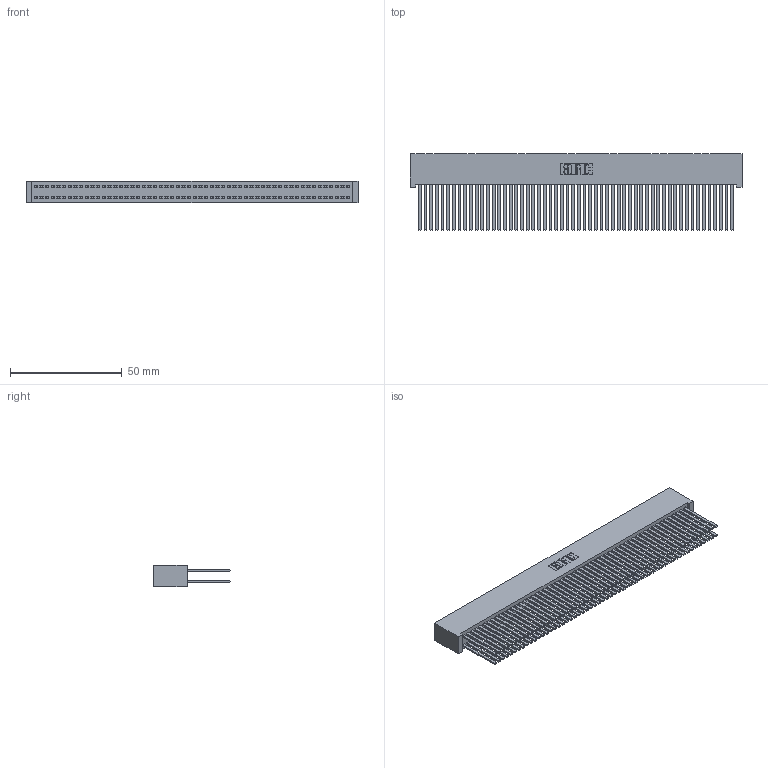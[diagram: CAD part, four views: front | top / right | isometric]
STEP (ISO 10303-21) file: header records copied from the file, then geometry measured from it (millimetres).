
FILE_DESCRIPTION (( 'STEP AP203' ), '1' );
FILE_NAME ('342-112-544-201.STEP', '2018-08-14T12:18:39', ( '' ), ( '' ), 'SwSTEP 2.0', 'SolidWorks 2016', '' );
FILE_SCHEMA (( 'CONFIG_CONTROL_DESIGN' ));
Length unit declared in the file: inch
Products named in the file (3): 345-292-001_345-293-144; 342-112-544-201; 342 Part_Lugless
Assembly tree (113 placements, depth 2):
  342-112-544-201
    342 Part_Lugless
    345-292-001_345-293-144  x112
Bounding box: 148.49 x 34.3 x 9.4 mm (x, y, z)
Volume: 15417.5 mm3; surface area: 30235 mm2
Topology: 113 solids, 113 shells, 5254 faces, 15619 edges, 10262 vertices
Faces by surface type: plane 3646, cylinder 1608
Entity records: 33623 total; most frequent: CARTESIAN_POINT 5550, ORIENTED_EDGE 5486, DIRECTION 4707, EDGE_CURVE 2743, VECTOR 2627, LINE 2627, VERTEX_POINT 1826, AXIS2_PLACEMENT_3D 1040
